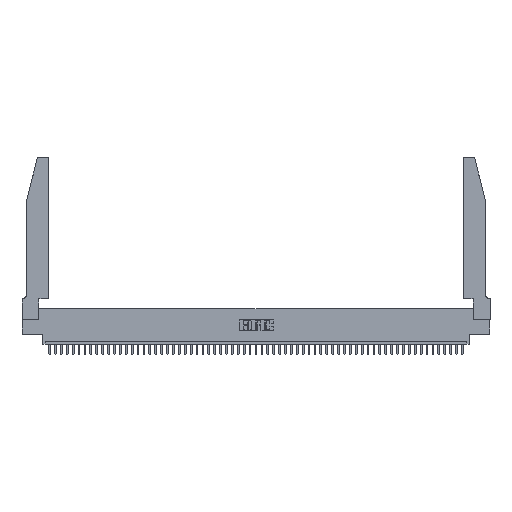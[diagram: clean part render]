
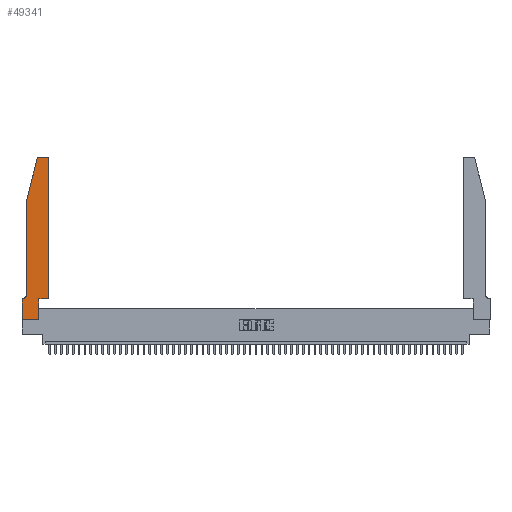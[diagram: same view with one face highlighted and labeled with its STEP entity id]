
A CAD part, top view. The second image highlights one B-rep face of the part: STEP entity #49341.
In plain terms, the highlighted planar face has unit normal (0, 0, 1).
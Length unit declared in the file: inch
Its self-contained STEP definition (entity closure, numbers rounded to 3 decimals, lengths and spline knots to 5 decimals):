
#516 = LINE ( 'NONE', #48244, #11130 ) ;
#608 = DIRECTION ( 'NONE',  ( -1., 0., 0. ) ) ;
#772 = CARTESIAN_POINT ( 'NONE',  ( 0.0755, 2., 0.37 ) ) ;
#1245 = CARTESIAN_POINT ( 'NONE',  ( 0., 0., 0.37 ) ) ;
#1334 = EDGE_CURVE ( 'NONE', #36880, #34874, #42093, .T. ) ;
#2437 = CARTESIAN_POINT ( 'NONE',  ( 0.25487, 2.72718, 0.37 ) ) ;
#3567 = AXIS2_PLACEMENT_3D ( 'NONE', #53171, #15270, #44330 ) ;
#4584 = ORIENTED_EDGE ( 'NONE', *, *, #51281, .T. ) ;
#5644 = DIRECTION ( 'NONE',  ( -0.239, -0.971, 0. ) ) ;
#5658 = DIRECTION ( 'NONE',  ( -1., 0., 0. ) ) ;
#6574 = LINE ( 'NONE', #40896, #27586 ) ;
#7503 = CARTESIAN_POINT ( 'NONE',  ( 0.4505, 0.35, 0.37 ) ) ;
#8151 = VERTEX_POINT ( 'NONE', #35816 ) ;
#8482 = VECTOR ( 'NONE', #50861, 39.37008 ) ;
#8747 = DIRECTION ( 'NONE',  ( 0., -1., 0. ) ) ;
#9274 = LINE ( 'NONE', #30853, #13221 ) ;
#9361 = LINE ( 'NONE', #42666, #52814 ) ;
#9590 = ORIENTED_EDGE ( 'NONE', *, *, #20963, .T. ) ;
#10115 = LINE ( 'NONE', #1245, #31866 ) ;
#10813 = CARTESIAN_POINT ( 'NONE',  ( 0.284, 2.75, 0.37 ) ) ;
#10926 = VERTEX_POINT ( 'NONE', #15002 ) ;
#11130 = VECTOR ( 'NONE', #38958, 39.37008 ) ;
#11520 = EDGE_CURVE ( 'NONE', #10926, #13021, #516, .T. ) ;
#11560 = CIRCLE ( 'NONE', #51348, 0.03 ) ;
#12583 = VERTEX_POINT ( 'NONE', #42176 ) ;
#13021 = VERTEX_POINT ( 'NONE', #44993 ) ;
#13221 = VECTOR ( 'NONE', #5644, 39.37008 ) ;
#14926 = DIRECTION ( 'NONE',  ( 1., 0., 0. ) ) ;
#15002 = CARTESIAN_POINT ( 'NONE',  ( 0.2865, 0., 0.37 ) ) ;
#15270 = DIRECTION ( 'NONE',  ( 0., 0., 1. ) ) ;
#16977 = EDGE_CURVE ( 'NONE', #28718, #10926, #10115, .T. ) ;
#16999 = ORIENTED_EDGE ( 'NONE', *, *, #38497, .T. ) ;
#17098 = LINE ( 'NONE', #54399, #19000 ) ;
#18611 = DIRECTION ( 'NONE',  ( 1., 0., 0. ) ) ;
#18698 = ORIENTED_EDGE ( 'NONE', *, *, #22172, .T. ) ;
#18875 = ORIENTED_EDGE ( 'NONE', *, *, #51604, .T. ) ;
#18909 = CARTESIAN_POINT ( 'NONE',  ( 0.0055, 0.42, 0.37 ) ) ;
#19000 = VECTOR ( 'NONE', #8747, 39.37008 ) ;
#19388 = ORIENTED_EDGE ( 'NONE', *, *, #1334, .T. ) ;
#19741 = DIRECTION ( 'NONE',  ( -1., 0., 0. ) ) ;
#20560 = DIRECTION ( 'NONE',  ( 1., 0., 0. ) ) ;
#20910 = CARTESIAN_POINT ( 'NONE',  ( 0.284, 2.72, 0.37 ) ) ;
#20963 = EDGE_CURVE ( 'NONE', #48735, #47287, #37369, .T. ) ;
#22172 = EDGE_CURVE ( 'NONE', #52106, #36880, #9274, .T. ) ;
#22735 = ORIENTED_EDGE ( 'NONE', *, *, #11520, .T. ) ;
#24343 = VECTOR ( 'NONE', #608, 39.37008 ) ;
#25103 = DIRECTION ( 'NONE',  ( 1., 0., 0. ) ) ;
#25367 = ORIENTED_EDGE ( 'NONE', *, *, #44964, .T. ) ;
#25748 = FACE_OUTER_BOUND ( 'NONE', #51753, .T. ) ;
#26683 = ORIENTED_EDGE ( 'NONE', *, *, #36600, .T. ) ;
#27586 = VECTOR ( 'NONE', #19741, 39.37008 ) ;
#28718 = VERTEX_POINT ( 'NONE', #32244 ) ;
#29355 = CARTESIAN_POINT ( 'NONE',  ( 0.0755, 2., 0.37 ) ) ;
#29453 = AXIS2_PLACEMENT_3D ( 'NONE', #18909, #35833, #5658 ) ;
#29818 = VERTEX_POINT ( 'NONE', #10813 ) ;
#29978 = EDGE_CURVE ( 'NONE', #12583, #48735, #9361, .T. ) ;
#30121 = DIRECTION ( 'NONE',  ( 0., 1., 0. ) ) ;
#30853 = CARTESIAN_POINT ( 'NONE',  ( 0.0755, 2., 0.37 ) ) ;
#31254 = CARTESIAN_POINT ( 'NONE',  ( 0.0755, 0.42, 0.37 ) ) ;
#31699 = PLANE ( 'NONE',  #32300 ) ;
#31866 = VECTOR ( 'NONE', #14926, 39.37008 ) ;
#32188 = ORIENTED_EDGE ( 'NONE', *, *, #16977, .T. ) ;
#32244 = CARTESIAN_POINT ( 'NONE',  ( 0., 0., 0.37 ) ) ;
#32300 = AXIS2_PLACEMENT_3D ( 'NONE', #48624, #44589, #18611 ) ;
#34874 = VERTEX_POINT ( 'NONE', #31254 ) ;
#35816 = CARTESIAN_POINT ( 'NONE',  ( 0., 0.35, 0.37 ) ) ;
#35833 = DIRECTION ( 'NONE',  ( 0., 0., -1. ) ) ;
#36355 = CARTESIAN_POINT ( 'NONE',  ( 0.4505, 2.72, 0.37 ) ) ;
#36600 = EDGE_CURVE ( 'NONE', #47287, #29818, #6574, .T. ) ;
#36880 = VERTEX_POINT ( 'NONE', #772 ) ;
#37369 = CIRCLE ( 'NONE', #3567, 0.03 ) ;
#38098 = LINE ( 'NONE', #7503, #40049 ) ;
#38497 = EDGE_CURVE ( 'NONE', #34874, #39633, #45338, .T. ) ;
#38958 = DIRECTION ( 'NONE',  ( 0., 1., 0. ) ) ;
#39429 = LINE ( 'NONE', #47592, #24343 ) ;
#39633 = VERTEX_POINT ( 'NONE', #43482 ) ;
#40049 = VECTOR ( 'NONE', #20560, 39.37008 ) ;
#40896 = CARTESIAN_POINT ( 'NONE',  ( 0.2605, 2.75, 0.37 ) ) ;
#41122 = CARTESIAN_POINT ( 'NONE',  ( 0.4205, 2.75, 0.37 ) ) ;
#41277 = EDGE_CURVE ( 'NONE', #29818, #52106, #11560, .T. ) ;
#42093 = LINE ( 'NONE', #29355, #8482 ) ;
#42176 = CARTESIAN_POINT ( 'NONE',  ( 0.4505, 0.35, 0.37 ) ) ;
#42666 = CARTESIAN_POINT ( 'NONE',  ( 0.4505, 0.35, 0.37 ) ) ;
#43482 = CARTESIAN_POINT ( 'NONE',  ( 0.0055, 0.35, 0.37 ) ) ;
#44330 = DIRECTION ( 'NONE',  ( 1., 0., 0. ) ) ;
#44589 = DIRECTION ( 'NONE',  ( 0., 0., 1. ) ) ;
#44964 = EDGE_CURVE ( 'NONE', #8151, #28718, #17098, .T. ) ;
#44993 = CARTESIAN_POINT ( 'NONE',  ( 0.2865, 0.35, 0.37 ) ) ;
#45338 = CIRCLE ( 'NONE', #29453, 0.07 ) ;
#46928 = ORIENTED_EDGE ( 'NONE', *, *, #29978, .T. ) ;
#47287 = VERTEX_POINT ( 'NONE', #41122 ) ;
#47592 = CARTESIAN_POINT ( 'NONE',  ( 0.0755, 0.35, 0.37 ) ) ;
#48244 = CARTESIAN_POINT ( 'NONE',  ( 0.2865, 0.35, 0.37 ) ) ;
#48624 = CARTESIAN_POINT ( 'NONE',  ( 0., 0.35, 0.37 ) ) ;
#48735 = VERTEX_POINT ( 'NONE', #36355 ) ;
#49109 = ORIENTED_EDGE ( 'NONE', *, *, #41277, .T. ) ;
#49341 = ADVANCED_FACE ( 'NONE', ( #25748 ), #31699, .T. ) ;
#50349 = DIRECTION ( 'NONE',  ( 0., 0., 1. ) ) ;
#50861 = DIRECTION ( 'NONE',  ( 0., -1., 0. ) ) ;
#51281 = EDGE_CURVE ( 'NONE', #39633, #8151, #39429, .T. ) ;
#51348 = AXIS2_PLACEMENT_3D ( 'NONE', #20910, #50349, #25103 ) ;
#51604 = EDGE_CURVE ( 'NONE', #13021, #12583, #38098, .T. ) ;
#51753 = EDGE_LOOP ( 'NONE', ( #26683, #49109, #18698, #19388, #16999, #4584, #25367, #32188, #22735, #18875, #46928, #9590 ) ) ;
#52106 = VERTEX_POINT ( 'NONE', #2437 ) ;
#52814 = VECTOR ( 'NONE', #30121, 39.37008 ) ;
#53171 = CARTESIAN_POINT ( 'NONE',  ( 0.4205, 2.72, 0.37 ) ) ;
#54399 = CARTESIAN_POINT ( 'NONE',  ( 0., 0., 0.37 ) ) ;
